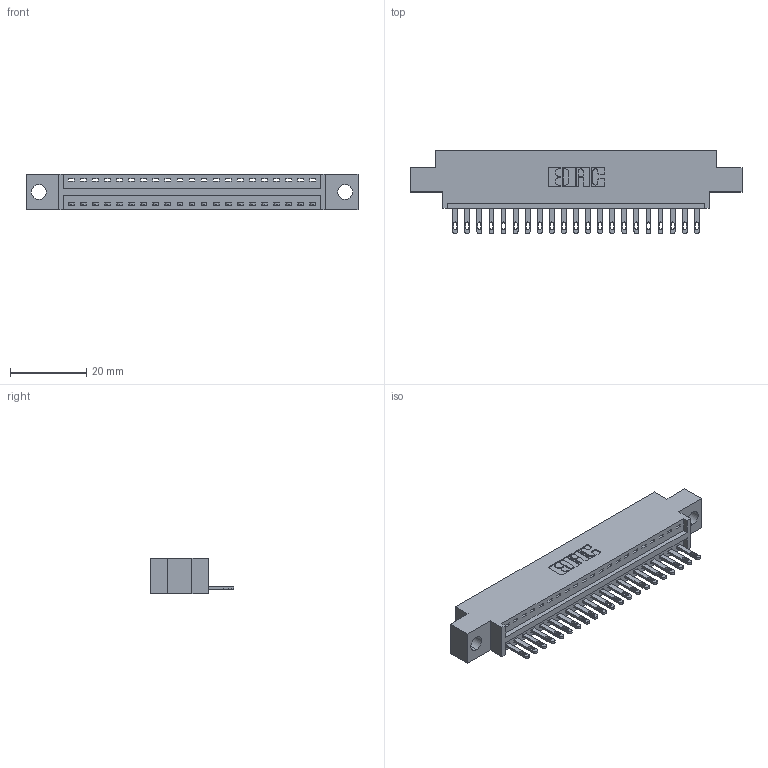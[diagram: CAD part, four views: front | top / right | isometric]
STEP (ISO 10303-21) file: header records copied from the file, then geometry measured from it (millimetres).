
FILE_DESCRIPTION (( 'STEP AP203' ), '1' );
FILE_NAME ('346-021-500-604.STEP', '2022-05-05T17:28:44', ( '' ), ( '' ), 'SwSTEP 2.0', 'SolidWorks 2020', '' );
FILE_SCHEMA (( 'CONFIG_CONTROL_DESIGN' ));
Length unit declared in the file: inch
Products named in the file (3): 345-292-001_345-293-100; 346-021-500-604; 346 Part_0.170 Offset - 0.156 Dia-TH
Assembly tree (22 placements, depth 2):
  346-021-500-604
    346 Part_0.170 Offset - 0.156 Dia-TH
    345-292-001_345-293-100  x21
Bounding box: 87.25 x 21.84 x 9.4 mm (x, y, z)
Volume: 7959.4 mm3; surface area: 9768.2 mm2
Topology: 22 solids, 22 shells, 1274 faces, 3905 edges, 2602 vertices
Faces by surface type: plane 808, cylinder 466
Entity records: 16341 total; most frequent: CARTESIAN_POINT 2817, ORIENTED_EDGE 2770, DIRECTION 2511, EDGE_CURVE 1385, VECTOR 1165, LINE 1165, VERTEX_POINT 922, AXIS2_PLACEMENT_3D 673
